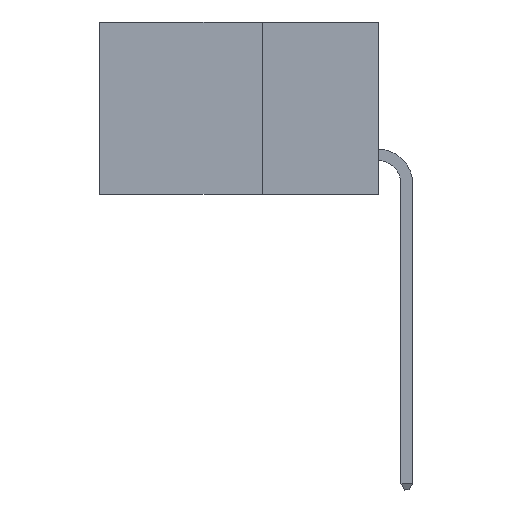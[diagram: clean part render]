
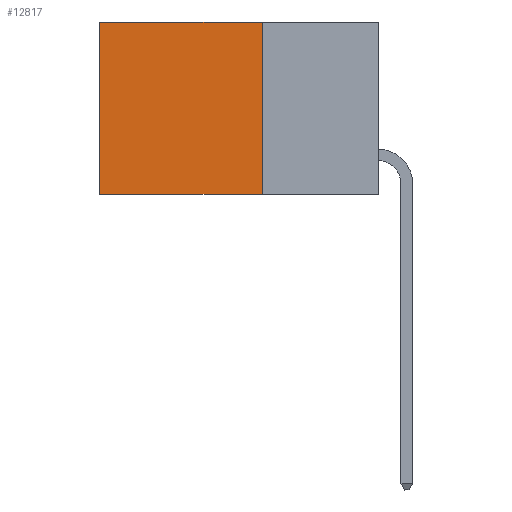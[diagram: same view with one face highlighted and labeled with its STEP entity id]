
A CAD part, left-side view. The second image highlights one B-rep face of the part: STEP entity #12817.
In plain terms, the highlighted planar face has unit normal (-1, 0, 0).
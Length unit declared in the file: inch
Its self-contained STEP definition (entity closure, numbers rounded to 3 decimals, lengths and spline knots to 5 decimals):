
#727 = CARTESIAN_POINT ( 'NONE',  ( 0.2615, 0.25, -0.37 ) ) ;
#982 = LINE ( 'NONE', #8544, #10605 ) ;
#1513 = DIRECTION ( 'NONE',  ( 0., 0., -1. ) ) ;
#3090 = ORIENTED_EDGE ( 'NONE', *, *, #23024, .F. ) ;
#4458 = AXIS2_PLACEMENT_3D ( 'NONE', #24173, #12963, #1513 ) ;
#4570 = LINE ( 'NONE', #19050, #14072 ) ;
#6196 = CARTESIAN_POINT ( 'NONE',  ( 0.2615, 0.25, 0. ) ) ;
#6212 = EDGE_CURVE ( 'NONE', #14998, #16054, #19111, .T. ) ;
#6316 = EDGE_CURVE ( 'NONE', #11266, #6600, #982, .T. ) ;
#6600 = VERTEX_POINT ( 'NONE', #16846 ) ;
#7652 = EDGE_LOOP ( 'NONE', ( #17914, #9547, #3090, #24134 ) ) ;
#8139 = EDGE_CURVE ( 'NONE', #16054, #6600, #4570, .T. ) ;
#8540 = VECTOR ( 'NONE', #15707, 39.37008 ) ;
#8544 = CARTESIAN_POINT ( 'NONE',  ( 0.2615, 0.25, -0.37 ) ) ;
#9547 = ORIENTED_EDGE ( 'NONE', *, *, #6316, .F. ) ;
#10436 = DIRECTION ( 'NONE',  ( 0., 1., 0. ) ) ;
#10605 = VECTOR ( 'NONE', #10436, 39.37008 ) ;
#11266 = VERTEX_POINT ( 'NONE', #18059 ) ;
#12203 = DIRECTION ( 'NONE',  ( 0., 0., -1. ) ) ;
#12817 = ADVANCED_FACE ( 'NONE', ( #15308 ), #12880, .F. ) ;
#12880 = PLANE ( 'NONE',  #4458 ) ;
#12963 = DIRECTION ( 'NONE',  ( 1., 0., 0. ) ) ;
#13513 = DIRECTION ( 'NONE',  ( 0., 0., -1. ) ) ;
#13931 = CARTESIAN_POINT ( 'NONE',  ( 0.2615, 0.25, 0. ) ) ;
#14072 = VECTOR ( 'NONE', #13513, 39.37008 ) ;
#14998 = VERTEX_POINT ( 'NONE', #13931 ) ;
#15308 = FACE_OUTER_BOUND ( 'NONE', #7652, .T. ) ;
#15707 = DIRECTION ( 'NONE',  ( 0., 1., 0. ) ) ;
#16054 = VERTEX_POINT ( 'NONE', #18780 ) ;
#16846 = CARTESIAN_POINT ( 'NONE',  ( 0.2615, 0.6, -0.37 ) ) ;
#17914 = ORIENTED_EDGE ( 'NONE', *, *, #8139, .T. ) ;
#18059 = CARTESIAN_POINT ( 'NONE',  ( 0.2615, 0.25, -0.37 ) ) ;
#18780 = CARTESIAN_POINT ( 'NONE',  ( 0.2615, 0.6, 0. ) ) ;
#18915 = VECTOR ( 'NONE', #12203, 39.37008 ) ;
#19050 = CARTESIAN_POINT ( 'NONE',  ( 0.2615, 0.6, -0.37 ) ) ;
#19111 = LINE ( 'NONE', #6196, #8540 ) ;
#23024 = EDGE_CURVE ( 'NONE', #14998, #11266, #24465, .T. ) ;
#24134 = ORIENTED_EDGE ( 'NONE', *, *, #6212, .T. ) ;
#24173 = CARTESIAN_POINT ( 'NONE',  ( 0.2615, 0.25, -0.37 ) ) ;
#24465 = LINE ( 'NONE', #727, #18915 ) ;
